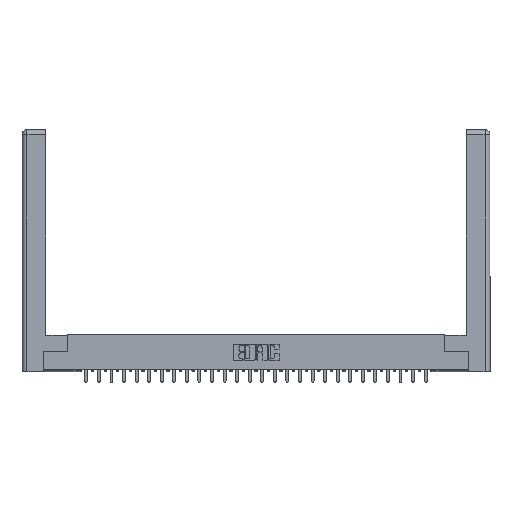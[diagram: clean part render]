
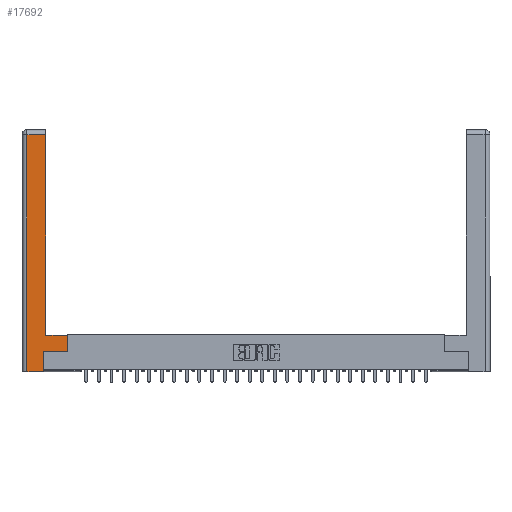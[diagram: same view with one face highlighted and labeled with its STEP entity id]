
A CAD part, top view. The second image highlights one B-rep face of the part: STEP entity #17692.
In plain terms, the highlighted planar face has unit normal (0, 0, 1).
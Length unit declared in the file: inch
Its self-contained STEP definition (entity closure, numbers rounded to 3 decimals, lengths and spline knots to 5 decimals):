
#2152 = CARTESIAN_POINT ( 'NONE',  ( 0., 0., 0. ) ) ;
#2210 = VECTOR ( 'NONE', #24656, 39.37008 ) ;
#2244 = LINE ( 'NONE', #10057, #14135 ) ;
#2336 = VERTEX_POINT ( 'NONE', #23902 ) ;
#2616 = ORIENTED_EDGE ( 'NONE', *, *, #15803, .T. ) ;
#2873 = FACE_OUTER_BOUND ( 'NONE', #28958, .T. ) ;
#2978 = LINE ( 'NONE', #3380, #2210 ) ;
#3064 = EDGE_CURVE ( 'NONE', #2336, #16533, #2244, .T. ) ;
#3380 = CARTESIAN_POINT ( 'NONE',  ( 0.265, 0., 0. ) ) ;
#3485 = EDGE_CURVE ( 'NONE', #14980, #10238, #2978, .T. ) ;
#3626 = ORIENTED_EDGE ( 'NONE', *, *, #3064, .T. ) ;
#3958 = DIRECTION ( 'NONE',  ( 0., 1., 0. ) ) ;
#4276 = LINE ( 'NONE', #11692, #22306 ) ;
#4553 = DIRECTION ( 'NONE',  ( -1., 0., 0. ) ) ;
#4795 = EDGE_CURVE ( 'NONE', #18537, #24456, #15551, .T. ) ;
#6162 = DIRECTION ( 'NONE',  ( 0., 1., 0. ) ) ;
#6270 = CARTESIAN_POINT ( 'NONE',  ( 0.0615, 0., 0. ) ) ;
#6461 = DIRECTION ( 'NONE',  ( -1., 0., 0. ) ) ;
#7600 = CARTESIAN_POINT ( 'NONE',  ( 0.265, 0.245, 0. ) ) ;
#7885 = AXIS2_PLACEMENT_3D ( 'NONE', #2152, #18724, #4553 ) ;
#9190 = VECTOR ( 'NONE', #22227, 39.37008 ) ;
#9669 = VERTEX_POINT ( 'NONE', #23699 ) ;
#9738 = ORIENTED_EDGE ( 'NONE', *, *, #27163, .T. ) ;
#9954 = DIRECTION ( 'NONE',  ( 0., 1., 0. ) ) ;
#10057 = CARTESIAN_POINT ( 'NONE',  ( 0.0615, 2.94, 0. ) ) ;
#10238 = VERTEX_POINT ( 'NONE', #28140 ) ;
#10603 = ORIENTED_EDGE ( 'NONE', *, *, #4795, .T. ) ;
#11259 = CARTESIAN_POINT ( 'NONE',  ( 0.565, 0.45, 0. ) ) ;
#11692 = CARTESIAN_POINT ( 'NONE',  ( 0.295, 0.45, 0. ) ) ;
#12282 = VECTOR ( 'NONE', #3958, 39.37008 ) ;
#13021 = VECTOR ( 'NONE', #6162, 39.37008 ) ;
#13100 = VERTEX_POINT ( 'NONE', #11259 ) ;
#14135 = VECTOR ( 'NONE', #6461, 39.37008 ) ;
#14608 = CARTESIAN_POINT ( 'NONE',  ( 0.0615, 0., 0. ) ) ;
#14980 = VERTEX_POINT ( 'NONE', #14608 ) ;
#15551 = LINE ( 'NONE', #23386, #9190 ) ;
#15764 = EDGE_CURVE ( 'NONE', #9669, #2336, #25408, .T. ) ;
#15803 = EDGE_CURVE ( 'NONE', #24456, #13100, #29413, .T. ) ;
#16403 = PLANE ( 'NONE',  #7885 ) ;
#16533 = VERTEX_POINT ( 'NONE', #18501 ) ;
#16705 = DIRECTION ( 'NONE',  ( -1., 0., 0. ) ) ;
#17692 = ADVANCED_FACE ( 'NONE', ( #2873 ), #16403, .F. ) ;
#18152 = CARTESIAN_POINT ( 'NONE',  ( 0.565, 0.45, 0. ) ) ;
#18501 = CARTESIAN_POINT ( 'NONE',  ( 0.0615, 2.94, 0. ) ) ;
#18537 = VERTEX_POINT ( 'NONE', #20001 ) ;
#18724 = DIRECTION ( 'NONE',  ( 0., 0., -1. ) ) ;
#20001 = CARTESIAN_POINT ( 'NONE',  ( 0.265, 0.245, 0. ) ) ;
#20251 = ORIENTED_EDGE ( 'NONE', *, *, #20504, .T. ) ;
#20465 = LINE ( 'NONE', #6270, #25147 ) ;
#20504 = EDGE_CURVE ( 'NONE', #10238, #18537, #22845, .T. ) ;
#21944 = ORIENTED_EDGE ( 'NONE', *, *, #3485, .T. ) ;
#22227 = DIRECTION ( 'NONE',  ( 1., 0., 0. ) ) ;
#22306 = VECTOR ( 'NONE', #16705, 39.37008 ) ;
#22663 = DIRECTION ( 'NONE',  ( 0., -1., 0. ) ) ;
#22845 = LINE ( 'NONE', #7600, #27569 ) ;
#23386 = CARTESIAN_POINT ( 'NONE',  ( 0.565, 0.245, 0. ) ) ;
#23699 = CARTESIAN_POINT ( 'NONE',  ( 0.295, 0.45, 0. ) ) ;
#23902 = CARTESIAN_POINT ( 'NONE',  ( 0.295, 2.94, 0. ) ) ;
#23970 = EDGE_CURVE ( 'NONE', #16533, #14980, #20465, .T. ) ;
#24456 = VERTEX_POINT ( 'NONE', #29053 ) ;
#24656 = DIRECTION ( 'NONE',  ( 1., 0., 0. ) ) ;
#25147 = VECTOR ( 'NONE', #22663, 39.37008 ) ;
#25408 = LINE ( 'NONE', #27154, #13021 ) ;
#26228 = ORIENTED_EDGE ( 'NONE', *, *, #15764, .T. ) ;
#26470 = ORIENTED_EDGE ( 'NONE', *, *, #23970, .T. ) ;
#27154 = CARTESIAN_POINT ( 'NONE',  ( 0.295, 3., 0. ) ) ;
#27163 = EDGE_CURVE ( 'NONE', #13100, #9669, #4276, .T. ) ;
#27569 = VECTOR ( 'NONE', #9954, 39.37008 ) ;
#28140 = CARTESIAN_POINT ( 'NONE',  ( 0.265, 0., 0. ) ) ;
#28958 = EDGE_LOOP ( 'NONE', ( #26228, #3626, #26470, #21944, #20251, #10603, #2616, #9738 ) ) ;
#29053 = CARTESIAN_POINT ( 'NONE',  ( 0.565, 0.245, 0. ) ) ;
#29413 = LINE ( 'NONE', #18152, #12282 ) ;
